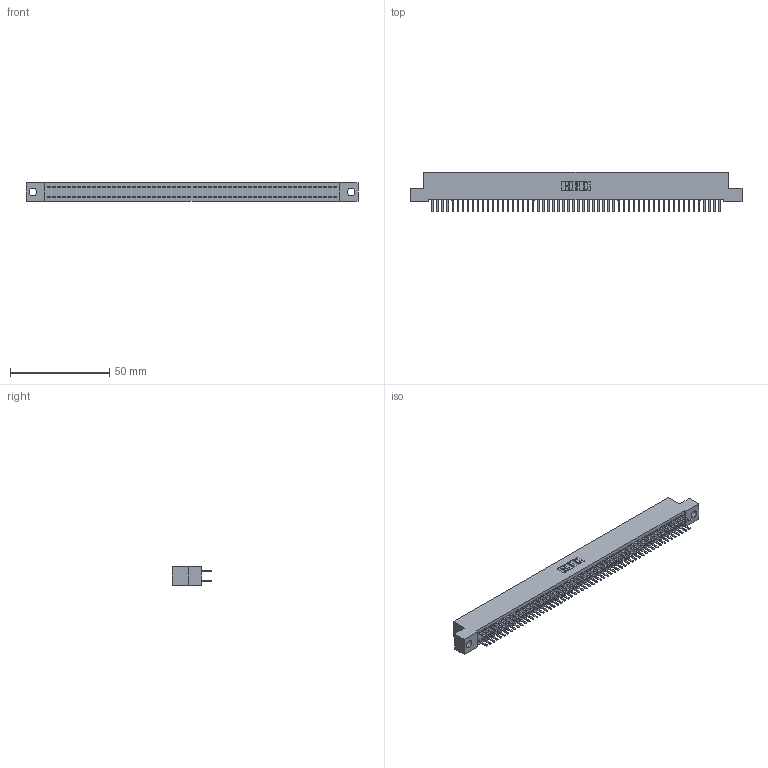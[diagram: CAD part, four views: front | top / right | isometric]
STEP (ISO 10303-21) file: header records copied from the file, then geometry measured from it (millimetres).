
FILE_DESCRIPTION (( 'STEP AP203' ), '1' );
FILE_NAME ('392-116-520-204.STEP', '2018-08-18T23:49:03', ( '' ), ( '' ), 'SwSTEP 2.0', 'SolidWorks 2016', '' );
FILE_SCHEMA (( 'CONFIG_CONTROL_DESIGN' ));
Length unit declared in the file: inch
Products named in the file (3): 342 Part_.156 TH; 345-292-001_345-293-120; 392-116-520-204
Assembly tree (117 placements, depth 2):
  392-116-520-204
    342 Part_.156 TH
    345-292-001_345-293-120  x116
Bounding box: 167.64 x 20.02 x 9.4 mm (x, y, z)
Volume: 15000.1 mm3; surface area: 24514.6 mm2
Topology: 117 solids, 117 shells, 6606 faces, 19207 edges, 12494 vertices
Faces by surface type: plane 4474, cylinder 2132
Entity records: 35229 total; most frequent: CARTESIAN_POINT 5830, ORIENTED_EDGE 5754, DIRECTION 4941, EDGE_CURVE 2877, VECTOR 2745, LINE 2745, VERTEX_POINT 1914, AXIS2_PLACEMENT_3D 1098
